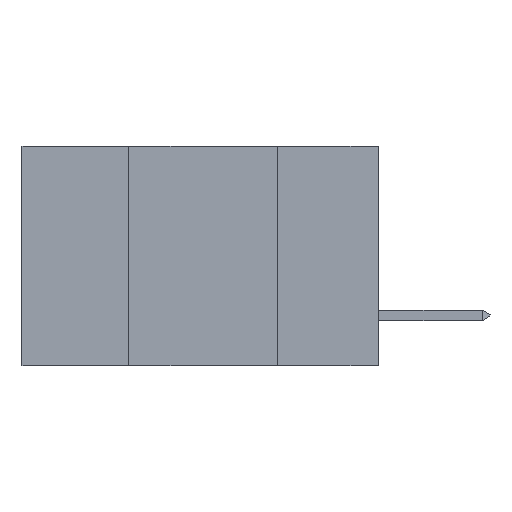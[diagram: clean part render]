
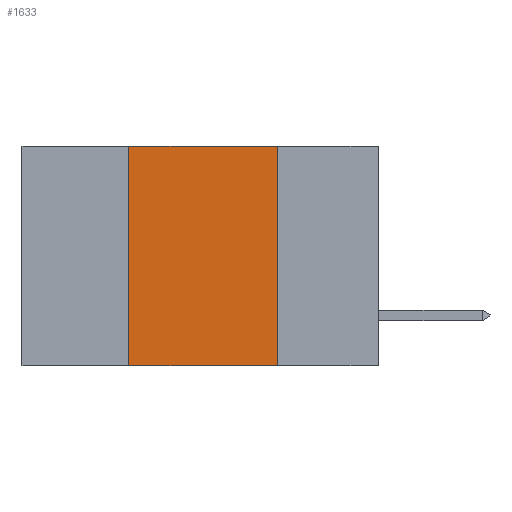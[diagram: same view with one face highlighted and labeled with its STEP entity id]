
A CAD part, left-side view. The second image highlights one B-rep face of the part: STEP entity #1633.
In plain terms, the highlighted planar face has unit normal (-1, 0, 0).
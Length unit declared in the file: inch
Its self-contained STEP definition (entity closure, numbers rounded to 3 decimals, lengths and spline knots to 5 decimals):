
#205 = VECTOR ( 'NONE', #6429, 39.37008 ) ;
#280 = CARTESIAN_POINT ( 'NONE',  ( 0., 0.42, 0. ) ) ;
#346 = LINE ( 'NONE', #5081, #10578 ) ;
#437 = DIRECTION ( 'NONE',  ( 0., 0., -1. ) ) ;
#1528 = CARTESIAN_POINT ( 'NONE',  ( 0., 0.17, 0. ) ) ;
#1633 = ADVANCED_FACE ( 'NONE', ( #8160 ), #13417, .F. ) ;
#1792 = DIRECTION ( 'NONE',  ( 0., 0., -1. ) ) ;
#2517 = ORIENTED_EDGE ( 'NONE', *, *, #13588, .F. ) ;
#2818 = ORIENTED_EDGE ( 'NONE', *, *, #12472, .T. ) ;
#2854 = ORIENTED_EDGE ( 'NONE', *, *, #5368, .F. ) ;
#3613 = DIRECTION ( 'NONE',  ( 1., 0., 0. ) ) ;
#3800 = VECTOR ( 'NONE', #1792, 39.37008 ) ;
#4280 = CARTESIAN_POINT ( 'NONE',  ( 0., 0.6, 0. ) ) ;
#5081 = CARTESIAN_POINT ( 'NONE',  ( 0., 0.42, -0.37 ) ) ;
#5368 = EDGE_CURVE ( 'NONE', #8245, #6193, #346, .T. ) ;
#6100 = CARTESIAN_POINT ( 'NONE',  ( 0., 0.42, -0.37 ) ) ;
#6164 = DIRECTION ( 'NONE',  ( 0., 0., 1. ) ) ;
#6193 = VERTEX_POINT ( 'NONE', #280 ) ;
#6283 = AXIS2_PLACEMENT_3D ( 'NONE', #11334, #3613, #437 ) ;
#6296 = EDGE_CURVE ( 'NONE', #10424, #7990, #12254, .T. ) ;
#6429 = DIRECTION ( 'NONE',  ( 0., -1., 0. ) ) ;
#6662 = CARTESIAN_POINT ( 'NONE',  ( 0., 0.17, -0.37 ) ) ;
#7086 = CARTESIAN_POINT ( 'NONE',  ( 0., 0.17, -0.37 ) ) ;
#7990 = VERTEX_POINT ( 'NONE', #6662 ) ;
#8160 = FACE_OUTER_BOUND ( 'NONE', #11969, .T. ) ;
#8245 = VERTEX_POINT ( 'NONE', #6100 ) ;
#8524 = DIRECTION ( 'NONE',  ( 0., -1., 0. ) ) ;
#8904 = VECTOR ( 'NONE', #8524, 39.37008 ) ;
#10424 = VERTEX_POINT ( 'NONE', #1528 ) ;
#10578 = VECTOR ( 'NONE', #6164, 39.37008 ) ;
#10725 = CARTESIAN_POINT ( 'NONE',  ( 0., 0.6, -0.37 ) ) ;
#11334 = CARTESIAN_POINT ( 'NONE',  ( 0., 0.6, 0. ) ) ;
#11657 = LINE ( 'NONE', #4280, #8904 ) ;
#11750 = LINE ( 'NONE', #10725, #205 ) ;
#11969 = EDGE_LOOP ( 'NONE', ( #13649, #2517, #2854, #2818 ) ) ;
#12254 = LINE ( 'NONE', #7086, #3800 ) ;
#12472 = EDGE_CURVE ( 'NONE', #8245, #7990, #11750, .T. ) ;
#13417 = PLANE ( 'NONE',  #6283 ) ;
#13588 = EDGE_CURVE ( 'NONE', #6193, #10424, #11657, .T. ) ;
#13649 = ORIENTED_EDGE ( 'NONE', *, *, #6296, .F. ) ;
